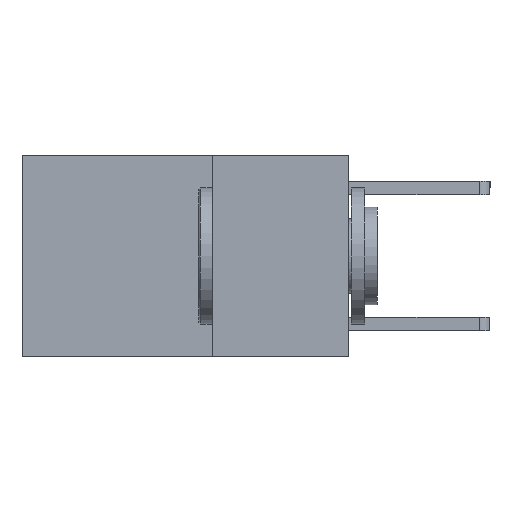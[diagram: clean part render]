
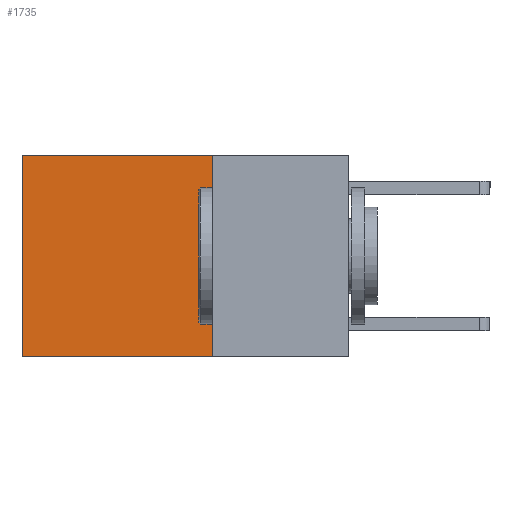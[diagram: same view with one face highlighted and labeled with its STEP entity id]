
A CAD part, left-side view. The second image highlights one B-rep face of the part: STEP entity #1735.
In plain terms, the highlighted planar face has unit normal (-1, 0, 0).
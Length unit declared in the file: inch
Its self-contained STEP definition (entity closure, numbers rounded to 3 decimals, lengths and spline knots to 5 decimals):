
#18 = VERTEX_POINT ( 'NONE', #2254 ) ;
#1044 = ORIENTED_EDGE ( 'NONE', *, *, #9338, .T. ) ;
#1735 = ADVANCED_FACE ( 'NONE', ( #5251 ), #2142, .F. ) ;
#1982 = DIRECTION ( 'NONE',  ( 1., 0., 0. ) ) ;
#2142 = PLANE ( 'NONE',  #9477 ) ;
#2238 = VECTOR ( 'NONE', #2374, 39.37008 ) ;
#2249 = EDGE_CURVE ( 'NONE', #6056, #6764, #7079, .T. ) ;
#2254 = CARTESIAN_POINT ( 'NONE',  ( 0.2625, 0.6, 0. ) ) ;
#2374 = DIRECTION ( 'NONE',  ( 0., 0., -1. ) ) ;
#3124 = DIRECTION ( 'NONE',  ( 0., 0., -1. ) ) ;
#3196 = CARTESIAN_POINT ( 'NONE',  ( 0.2625, 0.25, -0.37 ) ) ;
#3227 = EDGE_CURVE ( 'NONE', #6056, #18, #5989, .T. ) ;
#4122 = EDGE_CURVE ( 'NONE', #6764, #8610, #4921, .T. ) ;
#4921 = LINE ( 'NONE', #8128, #5669 ) ;
#5137 = DIRECTION ( 'NONE',  ( 0., 1., 0. ) ) ;
#5151 = EDGE_LOOP ( 'NONE', ( #1044, #7230, #9808, #7532 ) ) ;
#5251 = FACE_OUTER_BOUND ( 'NONE', #5151, .T. ) ;
#5653 = LINE ( 'NONE', #6394, #2238 ) ;
#5669 = VECTOR ( 'NONE', #7502, 39.37008 ) ;
#5989 = LINE ( 'NONE', #7605, #6522 ) ;
#6056 = VERTEX_POINT ( 'NONE', #7437 ) ;
#6394 = CARTESIAN_POINT ( 'NONE',  ( 0.2625, 0.6, 0. ) ) ;
#6522 = VECTOR ( 'NONE', #5137, 39.37008 ) ;
#6764 = VERTEX_POINT ( 'NONE', #3196 ) ;
#7079 = LINE ( 'NONE', #7961, #8145 ) ;
#7230 = ORIENTED_EDGE ( 'NONE', *, *, #4122, .F. ) ;
#7437 = CARTESIAN_POINT ( 'NONE',  ( 0.2625, 0.25, 0. ) ) ;
#7502 = DIRECTION ( 'NONE',  ( 0., 1., 0. ) ) ;
#7532 = ORIENTED_EDGE ( 'NONE', *, *, #3227, .T. ) ;
#7605 = CARTESIAN_POINT ( 'NONE',  ( 0.2625, 0.25, 0. ) ) ;
#7961 = CARTESIAN_POINT ( 'NONE',  ( 0.2625, 0.25, 0. ) ) ;
#8128 = CARTESIAN_POINT ( 'NONE',  ( 0.2625, 0.25, -0.37 ) ) ;
#8145 = VECTOR ( 'NONE', #3124, 39.37008 ) ;
#8402 = DIRECTION ( 'NONE',  ( 0., 0., -1. ) ) ;
#8610 = VERTEX_POINT ( 'NONE', #9184 ) ;
#9184 = CARTESIAN_POINT ( 'NONE',  ( 0.2625, 0.6, -0.37 ) ) ;
#9192 = CARTESIAN_POINT ( 'NONE',  ( 0.2625, 0.25, 0. ) ) ;
#9338 = EDGE_CURVE ( 'NONE', #18, #8610, #5653, .T. ) ;
#9477 = AXIS2_PLACEMENT_3D ( 'NONE', #9192, #1982, #8402 ) ;
#9808 = ORIENTED_EDGE ( 'NONE', *, *, #2249, .F. ) ;
